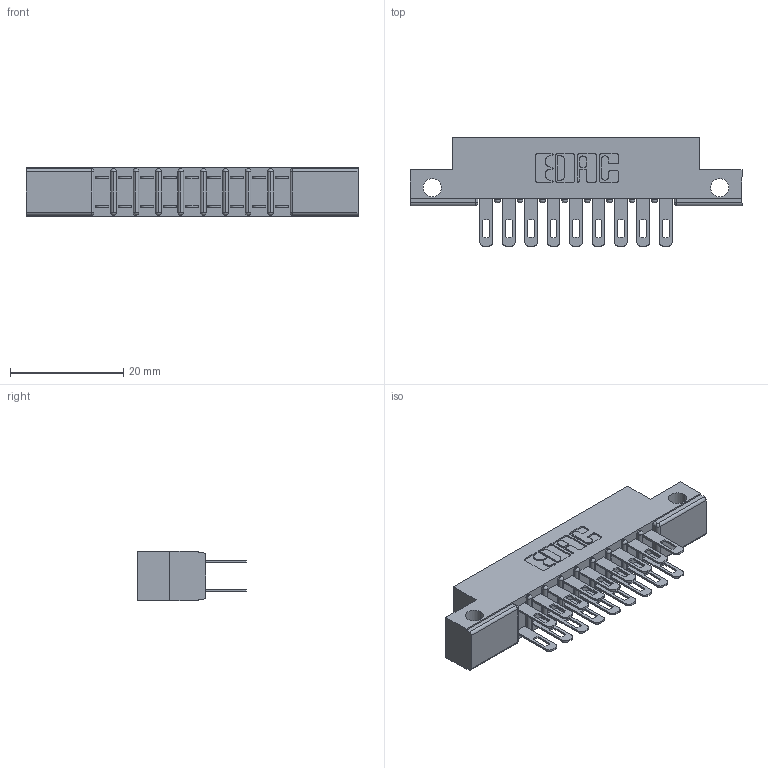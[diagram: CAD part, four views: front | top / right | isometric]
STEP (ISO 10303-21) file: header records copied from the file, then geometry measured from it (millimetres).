
FILE_DESCRIPTION (( 'STEP AP203' ), '1' );
FILE_NAME ('357-018-500-212.STEP', '2019-09-17T19:37:37', ( '' ), ( '' ), 'SwSTEP 2.0', 'SolidWorks 2016', '' );
FILE_SCHEMA (( 'CONFIG_CONTROL_DESIGN' ));
Length unit declared in the file: inch
Products named in the file (3): 357-018-500-212; 307 Part_.128 Dia Side Mounting Holes; 307-290-001_500
Assembly tree (19 placements, depth 2):
  357-018-500-212
    307 Part_.128 Dia Side Mounting Holes
    307-290-001_500  x18
Bounding box: 58.67 x 19.18 x 8.71 mm (x, y, z)
Volume: 3815 mm3; surface area: 6208.2 mm2
Topology: 19 solids, 19 shells, 956 faces, 2663 edges, 1722 vertices
Faces by surface type: plane 610, cylinder 326, sphere 20
Entity records: 12048 total; most frequent: CARTESIAN_POINT 1977, ORIENTED_EDGE 1954, DIRECTION 1953, EDGE_CURVE 977, VECTOR 733, LINE 733, VERTEX_POINT 634, AXIS2_PLACEMENT_3D 610
